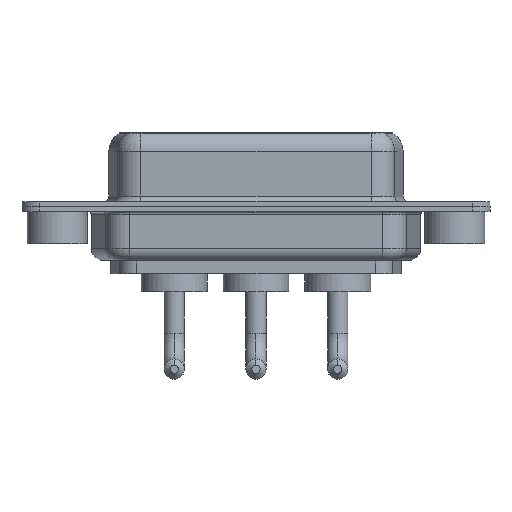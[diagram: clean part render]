
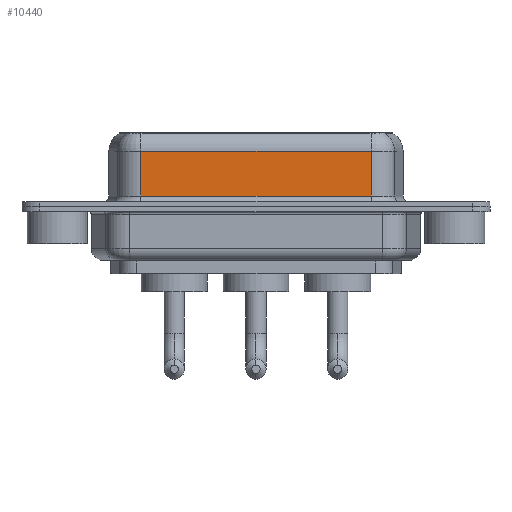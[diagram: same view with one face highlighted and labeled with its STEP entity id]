
A CAD part, front view. The second image highlights one B-rep face of the part: STEP entity #10440.
In plain terms, the highlighted planar face has unit normal (0, -1, 0).
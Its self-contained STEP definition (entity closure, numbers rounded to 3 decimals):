
#408 = CARTESIAN_POINT ( 'NONE',  ( 26.287, -3.95, 6.4 ) ) ;
#438 = EDGE_CURVE ( 'NONE', #11628, #4988, #4059, .T. ) ;
#507 = CARTESIAN_POINT ( 'NONE',  ( 26.287, -3.95, 4.65 ) ) ;
#641 = ORIENTED_EDGE ( 'NONE', *, *, #4145, .F. ) ;
#1047 = EDGE_CURVE ( 'NONE', #12260, #1103, #8219, .T. ) ;
#1103 = VERTEX_POINT ( 'NONE', #5612 ) ;
#1175 = ORIENTED_EDGE ( 'NONE', *, *, #438, .T. ) ;
#1633 = ORIENTED_EDGE ( 'NONE', *, *, #1683, .T. ) ;
#1683 = EDGE_CURVE ( 'NONE', #1103, #11628, #8368, .T. ) ;
#1765 = ORIENTED_EDGE ( 'NONE', *, *, #1047, .T. ) ;
#2041 = CARTESIAN_POINT ( 'NONE',  ( 7.013, -3.95, 0.9 ) ) ;
#3602 = AXIS2_PLACEMENT_3D ( 'NONE', #408, #6088, #11927 ) ;
#4059 = LINE ( 'NONE', #7857, #7386 ) ;
#4145 = EDGE_CURVE ( 'NONE', #12260, #4988, #6982, .T. ) ;
#4653 = CARTESIAN_POINT ( 'NONE',  ( 7.013, -3.95, 6.4 ) ) ;
#4848 = VECTOR ( 'NONE', #4871, 1000. ) ;
#4871 = DIRECTION ( 'NONE',  ( 0., 0., -1. ) ) ;
#4988 = VERTEX_POINT ( 'NONE', #10266 ) ;
#5269 = FACE_OUTER_BOUND ( 'NONE', #11916, .T. ) ;
#5612 = CARTESIAN_POINT ( 'NONE',  ( 7.013, -3.95, 4.65 ) ) ;
#5883 = CARTESIAN_POINT ( 'NONE',  ( 26.287, -3.95, 4.65 ) ) ;
#6088 = DIRECTION ( 'NONE',  ( 0., 1., 0. ) ) ;
#6865 = CARTESIAN_POINT ( 'NONE',  ( 26.287, -3.95, 6.4 ) ) ;
#6982 = LINE ( 'NONE', #6865, #4848 ) ;
#7386 = VECTOR ( 'NONE', #11654, 1000. ) ;
#7857 = CARTESIAN_POINT ( 'NONE',  ( 26.287, -3.95, 0.9 ) ) ;
#8219 = LINE ( 'NONE', #507, #10165 ) ;
#8368 = LINE ( 'NONE', #4653, #10947 ) ;
#10165 = VECTOR ( 'NONE', #10961, 1000. ) ;
#10266 = CARTESIAN_POINT ( 'NONE',  ( 26.287, -3.95, 0.9 ) ) ;
#10440 = ADVANCED_FACE ( 'NONE', ( #5269 ), #10923, .F. ) ;
#10923 = PLANE ( 'NONE',  #3602 ) ;
#10947 = VECTOR ( 'NONE', #12185, 1000. ) ;
#10961 = DIRECTION ( 'NONE',  ( -1., 0., 0. ) ) ;
#11628 = VERTEX_POINT ( 'NONE', #2041 ) ;
#11654 = DIRECTION ( 'NONE',  ( 1., 0., 0. ) ) ;
#11916 = EDGE_LOOP ( 'NONE', ( #641, #1765, #1633, #1175 ) ) ;
#11927 = DIRECTION ( 'NONE',  ( 0., 0., 1. ) ) ;
#12185 = DIRECTION ( 'NONE',  ( 0., 0., -1. ) ) ;
#12260 = VERTEX_POINT ( 'NONE', #5883 ) ;
